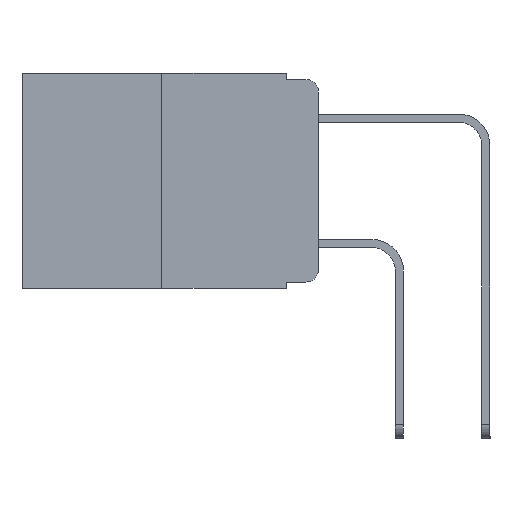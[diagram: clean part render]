
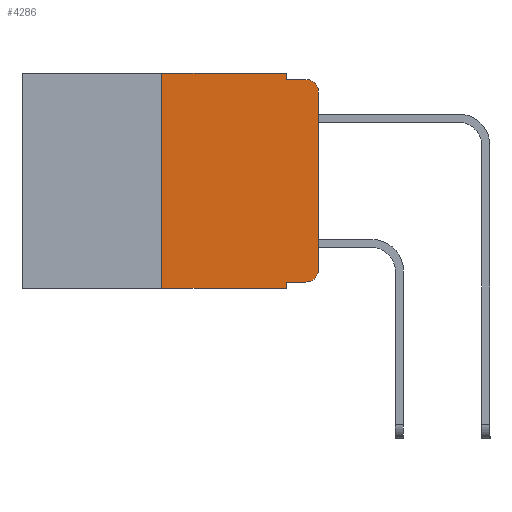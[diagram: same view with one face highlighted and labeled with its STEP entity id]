
A CAD part, left-side view. The second image highlights one B-rep face of the part: STEP entity #4286.
In plain terms, the highlighted planar face has unit normal (-1, 0, 0).
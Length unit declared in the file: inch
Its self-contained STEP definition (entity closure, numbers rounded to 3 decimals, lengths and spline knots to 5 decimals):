
#381 = VERTEX_POINT ( 'NONE', #4424 ) ;
#1280 = ORIENTED_EDGE ( 'NONE', *, *, #18688, .T. ) ;
#1359 = CARTESIAN_POINT ( 'NONE',  ( 0., 0.051, -0.01 ) ) ;
#2165 = DIRECTION ( 'NONE',  ( 0., 0., -1. ) ) ;
#2567 = ORIENTED_EDGE ( 'NONE', *, *, #19795, .T. ) ;
#2648 = EDGE_CURVE ( 'NONE', #8194, #11833, #22243, .T. ) ;
#3642 = VECTOR ( 'NONE', #23277, 39.37008 ) ;
#4075 = DIRECTION ( 'NONE',  ( -1., 0., 0. ) ) ;
#4286 = ADVANCED_FACE ( 'NONE', ( #6617 ), #7335, .F. ) ;
#4424 = CARTESIAN_POINT ( 'NONE',  ( 0., 0.02, -0.333 ) ) ;
#4884 = CARTESIAN_POINT ( 'NONE',  ( 0., 0.051, -0.343 ) ) ;
#5303 = EDGE_CURVE ( 'NONE', #381, #18726, #10866, .T. ) ;
#5321 = CARTESIAN_POINT ( 'NONE',  ( 0., 0.473, 0. ) ) ;
#5405 = CARTESIAN_POINT ( 'NONE',  ( 0., 0.25, -0.343 ) ) ;
#5865 = LINE ( 'NONE', #1359, #11659 ) ;
#5975 = ORIENTED_EDGE ( 'NONE', *, *, #24935, .F. ) ;
#6214 = DIRECTION ( 'NONE',  ( 0., -1., 0. ) ) ;
#6343 = CARTESIAN_POINT ( 'NONE',  ( 0., 0.051, -0.01 ) ) ;
#6617 = FACE_OUTER_BOUND ( 'NONE', #16467, .T. ) ;
#6988 = VERTEX_POINT ( 'NONE', #5405 ) ;
#7007 = VERTEX_POINT ( 'NONE', #22642 ) ;
#7335 = PLANE ( 'NONE',  #12981 ) ;
#7466 = VERTEX_POINT ( 'NONE', #8727 ) ;
#7840 = CARTESIAN_POINT ( 'NONE',  ( 0., 0.051, -0.333 ) ) ;
#8194 = VERTEX_POINT ( 'NONE', #20387 ) ;
#8403 = DIRECTION ( 'NONE',  ( -1., 0., 0. ) ) ;
#8641 = VERTEX_POINT ( 'NONE', #19796 ) ;
#8701 = LINE ( 'NONE', #24511, #23270 ) ;
#8713 = ORIENTED_EDGE ( 'NONE', *, *, #19976, .T. ) ;
#8727 = CARTESIAN_POINT ( 'NONE',  ( 0., 0.25, 0. ) ) ;
#9083 = DIRECTION ( 'NONE',  ( 0., 0., -1. ) ) ;
#9434 = DIRECTION ( 'NONE',  ( 0., 0., -1. ) ) ;
#9616 = ORIENTED_EDGE ( 'NONE', *, *, #21236, .F. ) ;
#10206 = EDGE_CURVE ( 'NONE', #7466, #8641, #18864, .T. ) ;
#10256 = AXIS2_PLACEMENT_3D ( 'NONE', #19864, #8403, #21760 ) ;
#10866 = CIRCLE ( 'NONE', #10256, 0.02 ) ;
#11659 = VECTOR ( 'NONE', #13089, 39.37008 ) ;
#11833 = VERTEX_POINT ( 'NONE', #4884 ) ;
#11873 = CARTESIAN_POINT ( 'NONE',  ( 0., 0., 0. ) ) ;
#12920 = VECTOR ( 'NONE', #15307, 39.37008 ) ;
#12981 = AXIS2_PLACEMENT_3D ( 'NONE', #5321, #18792, #9083 ) ;
#13089 = DIRECTION ( 'NONE',  ( 0., -1., 0. ) ) ;
#13212 = VECTOR ( 'NONE', #6214, 39.37008 ) ;
#13331 = DIRECTION ( 'NONE',  ( 0., 0., 1. ) ) ;
#13394 = LINE ( 'NONE', #11873, #3642 ) ;
#13647 = VERTEX_POINT ( 'NONE', #6343 ) ;
#14464 = VERTEX_POINT ( 'NONE', #16851 ) ;
#14503 = ORIENTED_EDGE ( 'NONE', *, *, #2648, .F. ) ;
#14609 = LINE ( 'NONE', #7840, #17857 ) ;
#15307 = DIRECTION ( 'NONE',  ( 0., -1., 0. ) ) ;
#15696 = CARTESIAN_POINT ( 'NONE',  ( 0., 0.02, -0.03 ) ) ;
#15729 = VECTOR ( 'NONE', #13331, 39.37008 ) ;
#15777 = AXIS2_PLACEMENT_3D ( 'NONE', #15696, #4075, #17595 ) ;
#15863 = CARTESIAN_POINT ( 'NONE',  ( 0., 0.473, 0. ) ) ;
#16467 = EDGE_LOOP ( 'NONE', ( #8713, #1280, #16827, #9616, #18305, #5975, #2567, #14503, #16479, #22771 ) ) ;
#16479 = ORIENTED_EDGE ( 'NONE', *, *, #23710, .T. ) ;
#16827 = ORIENTED_EDGE ( 'NONE', *, *, #22474, .F. ) ;
#16851 = CARTESIAN_POINT ( 'NONE',  ( 0., 0.02, -0.01 ) ) ;
#17312 = DIRECTION ( 'NONE',  ( 0., -1., 0. ) ) ;
#17595 = DIRECTION ( 'NONE',  ( 0., 0., -1. ) ) ;
#17857 = VECTOR ( 'NONE', #17312, 39.37008 ) ;
#18305 = ORIENTED_EDGE ( 'NONE', *, *, #10206, .F. ) ;
#18593 = CIRCLE ( 'NONE', #15777, 0.02 ) ;
#18688 = EDGE_CURVE ( 'NONE', #7007, #14464, #18593, .T. ) ;
#18726 = VERTEX_POINT ( 'NONE', #19584 ) ;
#18792 = DIRECTION ( 'NONE',  ( 1., 0., 0. ) ) ;
#18864 = LINE ( 'NONE', #15863, #13212 ) ;
#19584 = CARTESIAN_POINT ( 'NONE',  ( 0., 0., -0.313 ) ) ;
#19795 = EDGE_CURVE ( 'NONE', #6988, #11833, #23563, .T. ) ;
#19796 = CARTESIAN_POINT ( 'NONE',  ( 0., 0.051, 0. ) ) ;
#19864 = CARTESIAN_POINT ( 'NONE',  ( 0., 0.02, -0.313 ) ) ;
#19976 = EDGE_CURVE ( 'NONE', #18726, #7007, #13394, .T. ) ;
#20387 = CARTESIAN_POINT ( 'NONE',  ( 0., 0.051, -0.333 ) ) ;
#20925 = CARTESIAN_POINT ( 'NONE',  ( 0., 0.473, -0.343 ) ) ;
#21236 = EDGE_CURVE ( 'NONE', #8641, #13647, #8701, .T. ) ;
#21348 = LINE ( 'NONE', #24603, #15729 ) ;
#21760 = DIRECTION ( 'NONE',  ( 0., 0., -1. ) ) ;
#21939 = CARTESIAN_POINT ( 'NONE',  ( 0., 0.051, 0. ) ) ;
#22243 = LINE ( 'NONE', #21939, #23977 ) ;
#22474 = EDGE_CURVE ( 'NONE', #13647, #14464, #5865, .T. ) ;
#22642 = CARTESIAN_POINT ( 'NONE',  ( 0., 0., -0.03 ) ) ;
#22771 = ORIENTED_EDGE ( 'NONE', *, *, #5303, .T. ) ;
#23270 = VECTOR ( 'NONE', #9434, 39.37008 ) ;
#23277 = DIRECTION ( 'NONE',  ( 0., 0., 1. ) ) ;
#23563 = LINE ( 'NONE', #20925, #12920 ) ;
#23710 = EDGE_CURVE ( 'NONE', #8194, #381, #14609, .T. ) ;
#23977 = VECTOR ( 'NONE', #2165, 39.37008 ) ;
#24511 = CARTESIAN_POINT ( 'NONE',  ( 0., 0.051, 0. ) ) ;
#24603 = CARTESIAN_POINT ( 'NONE',  ( 0., 0.25, 0. ) ) ;
#24935 = EDGE_CURVE ( 'NONE', #6988, #7466, #21348, .T. ) ;
